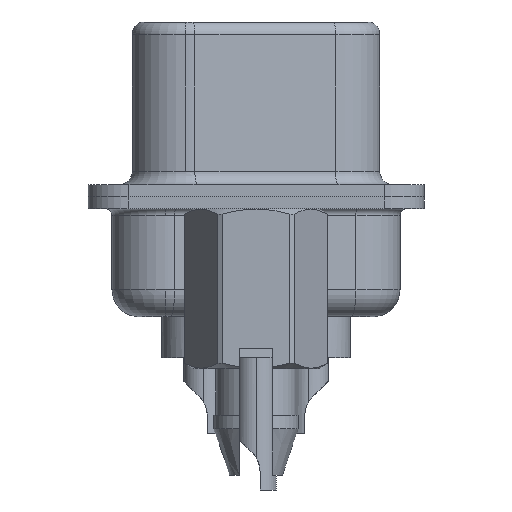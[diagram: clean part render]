
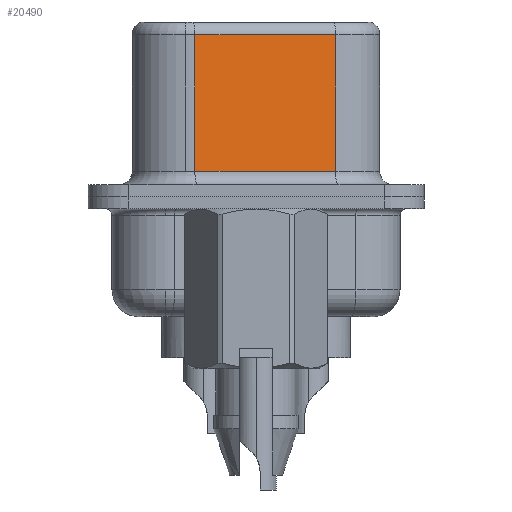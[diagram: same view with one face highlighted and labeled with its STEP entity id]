
A CAD part, left-side view. The second image highlights one B-rep face of the part: STEP entity #20490.
In plain terms, the highlighted planar face has unit normal (-0.985, -0.174, 0).
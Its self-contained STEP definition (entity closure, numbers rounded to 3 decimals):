
#213 = LINE ( 'NONE', #5974, #23474 ) ;
#1099 = ORIENTED_EDGE ( 'NONE', *, *, #24561, .T. ) ;
#2654 = DIRECTION ( 'NONE',  ( 0.174, -0.985, 0. ) ) ;
#4058 = DIRECTION ( 'NONE',  ( 0.985, 0.174, 0. ) ) ;
#5366 = ORIENTED_EDGE ( 'NONE', *, *, #12576, .T. ) ;
#5931 = CARTESIAN_POINT ( 'NONE',  ( 4.546, -2.987, 6.57 ) ) ;
#5962 = CARTESIAN_POINT ( 'NONE',  ( 4.546, -2.987, 0.95 ) ) ;
#5974 = CARTESIAN_POINT ( 'NONE',  ( 3.615, 2.293, 6.57 ) ) ;
#6284 = DIRECTION ( 'NONE',  ( -0.174, 0.985, 0. ) ) ;
#7154 = CARTESIAN_POINT ( 'NONE',  ( 3.615, 2.293, 6.07 ) ) ;
#7161 = CARTESIAN_POINT ( 'NONE',  ( 4.546, -2.987, 6.07 ) ) ;
#7745 = DIRECTION ( 'NONE',  ( 0., 0., -1. ) ) ;
#7951 = DIRECTION ( 'NONE',  ( -0.174, 0.985, 0. ) ) ;
#8165 = CARTESIAN_POINT ( 'NONE',  ( 4.546, -2.987, 0.95 ) ) ;
#8308 = LINE ( 'NONE', #14203, #23530 ) ;
#9949 = ORIENTED_EDGE ( 'NONE', *, *, #10483, .T. ) ;
#10483 = EDGE_CURVE ( 'NONE', #15247, #10901, #8308, .T. ) ;
#10901 = VERTEX_POINT ( 'NONE', #7154 ) ;
#11597 = CARTESIAN_POINT ( 'NONE',  ( 3.615, 2.293, 0.95 ) ) ;
#11764 = AXIS2_PLACEMENT_3D ( 'NONE', #5931, #4058, #7951 ) ;
#12576 = EDGE_CURVE ( 'NONE', #21667, #17805, #16071, .T. ) ;
#13982 = EDGE_CURVE ( 'NONE', #15247, #17805, #20591, .T. ) ;
#14203 = CARTESIAN_POINT ( 'NONE',  ( 4.546, -2.987, 6.07 ) ) ;
#14358 = VECTOR ( 'NONE', #2654, 1000. ) ;
#15205 = DIRECTION ( 'NONE',  ( 0., 0., -1. ) ) ;
#15247 = VERTEX_POINT ( 'NONE', #7161 ) ;
#15485 = PLANE ( 'NONE',  #11764 ) ;
#16071 = LINE ( 'NONE', #8165, #14358 ) ;
#17469 = FACE_OUTER_BOUND ( 'NONE', #20692, .T. ) ;
#17805 = VERTEX_POINT ( 'NONE', #5962 ) ;
#20137 = VECTOR ( 'NONE', #15205, 1000. ) ;
#20490 = ADVANCED_FACE ( 'NONE', ( #17469 ), #15485, .F. ) ;
#20591 = LINE ( 'NONE', #22733, #20137 ) ;
#20692 = EDGE_LOOP ( 'NONE', ( #22766, #9949, #1099, #5366 ) ) ;
#21667 = VERTEX_POINT ( 'NONE', #11597 ) ;
#22733 = CARTESIAN_POINT ( 'NONE',  ( 4.546, -2.987, 6.57 ) ) ;
#22766 = ORIENTED_EDGE ( 'NONE', *, *, #13982, .F. ) ;
#23474 = VECTOR ( 'NONE', #7745, 1000. ) ;
#23530 = VECTOR ( 'NONE', #6284, 1000. ) ;
#24561 = EDGE_CURVE ( 'NONE', #10901, #21667, #213, .T. ) ;
